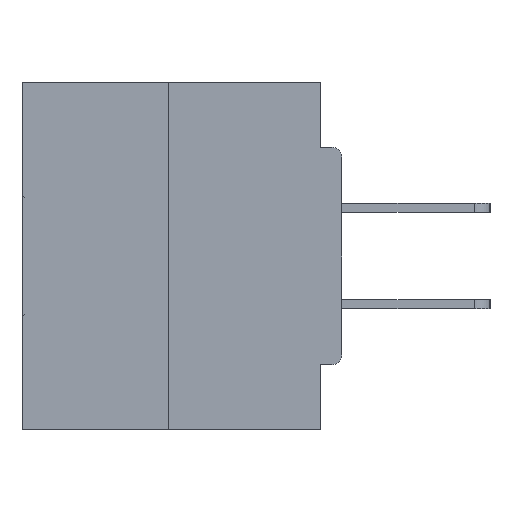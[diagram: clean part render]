
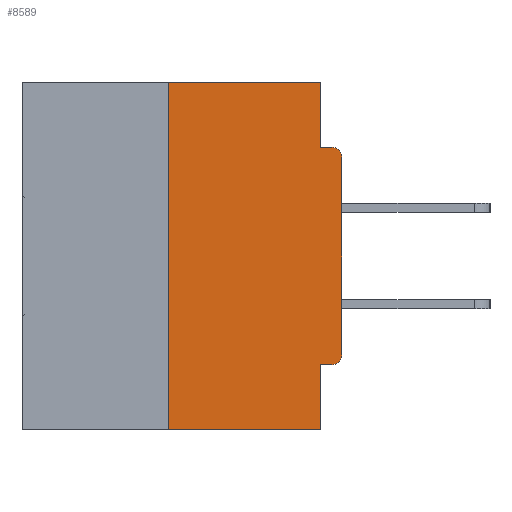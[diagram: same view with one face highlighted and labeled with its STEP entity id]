
A CAD part, left-side view. The second image highlights one B-rep face of the part: STEP entity #8589.
In plain terms, the highlighted planar face has unit normal (-1, 0, 0).
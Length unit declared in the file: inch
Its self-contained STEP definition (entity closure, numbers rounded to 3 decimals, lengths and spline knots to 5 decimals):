
#733 = LINE ( 'NONE', #10267, #17764 ) ;
#764 = VERTEX_POINT ( 'NONE', #37762 ) ;
#1586 = CARTESIAN_POINT ( 'NONE',  ( 0., 0., -0.3915 ) ) ;
#2046 = CARTESIAN_POINT ( 'NONE',  ( 0., 0., -0.0935 ) ) ;
#2396 = ORIENTED_EDGE ( 'NONE', *, *, #37040, .T. ) ;
#2832 = LINE ( 'NONE', #18832, #3875 ) ;
#3875 = VECTOR ( 'NONE', #12178, 39.37008 ) ;
#3882 = ORIENTED_EDGE ( 'NONE', *, *, #20483, .F. ) ;
#5641 = CARTESIAN_POINT ( 'NONE',  ( 0., 0.015, -0.1085 ) ) ;
#5888 = VERTEX_POINT ( 'NONE', #15403 ) ;
#6257 = DIRECTION ( 'NONE',  ( 0., 0., -1. ) ) ;
#7537 = LINE ( 'NONE', #38328, #28983 ) ;
#7588 = VERTEX_POINT ( 'NONE', #38716 ) ;
#7841 = VERTEX_POINT ( 'NONE', #35163 ) ;
#8545 = DIRECTION ( 'NONE',  ( 0., 0., 1. ) ) ;
#8589 = ADVANCED_FACE ( 'NONE', ( #15275 ), #27434, .F. ) ;
#8848 = EDGE_CURVE ( 'NONE', #7841, #5888, #20294, .T. ) ;
#9778 = DIRECTION ( 'NONE',  ( 0., 0., -1. ) ) ;
#10267 = CARTESIAN_POINT ( 'NONE',  ( 0., 0., 0. ) ) ;
#10651 = ORIENTED_EDGE ( 'NONE', *, *, #24445, .F. ) ;
#10843 = ORIENTED_EDGE ( 'NONE', *, *, #22817, .T. ) ;
#11865 = VERTEX_POINT ( 'NONE', #22563 ) ;
#12178 = DIRECTION ( 'NONE',  ( 0., 0., -1. ) ) ;
#12375 = CIRCLE ( 'NONE', #34982, 0.015 ) ;
#12980 = DIRECTION ( 'NONE',  ( 0., 0., -1. ) ) ;
#13214 = ORIENTED_EDGE ( 'NONE', *, *, #31585, .F. ) ;
#13827 = DIRECTION ( 'NONE',  ( 0., -1., 0. ) ) ;
#13880 = EDGE_LOOP ( 'NONE', ( #26750, #13214, #10843, #32011, #3882, #2396, #17291, #15382, #14777, #10651 ) ) ;
#13965 = EDGE_CURVE ( 'NONE', #7588, #19738, #7537, .T. ) ;
#14474 = VECTOR ( 'NONE', #31042, 39.37008 ) ;
#14777 = ORIENTED_EDGE ( 'NONE', *, *, #8848, .F. ) ;
#15275 = FACE_OUTER_BOUND ( 'NONE', #13880, .T. ) ;
#15382 = ORIENTED_EDGE ( 'NONE', *, *, #29497, .T. ) ;
#15403 = CARTESIAN_POINT ( 'NONE',  ( 0., 0.015, -0.0935 ) ) ;
#15843 = LINE ( 'NONE', #34251, #22243 ) ;
#16176 = VERTEX_POINT ( 'NONE', #1586 ) ;
#17291 = ORIENTED_EDGE ( 'NONE', *, *, #23806, .T. ) ;
#17660 = VECTOR ( 'NONE', #36075, 39.37008 ) ;
#17764 = VECTOR ( 'NONE', #31330, 39.37008 ) ;
#18023 = DIRECTION ( 'NONE',  ( 0., 0., -1. ) ) ;
#18832 = CARTESIAN_POINT ( 'NONE',  ( 0., 0.031, -0.5 ) ) ;
#19074 = VECTOR ( 'NONE', #6257, 39.37008 ) ;
#19128 = AXIS2_PLACEMENT_3D ( 'NONE', #5641, #32589, #18023 ) ;
#19738 = VERTEX_POINT ( 'NONE', #21620 ) ;
#20294 = LINE ( 'NONE', #2046, #17660 ) ;
#20327 = CARTESIAN_POINT ( 'NONE',  ( 0., 0.015, -0.4065 ) ) ;
#20483 = EDGE_CURVE ( 'NONE', #27282, #27131, #37099, .T. ) ;
#21620 = CARTESIAN_POINT ( 'NONE',  ( 0., 0.031, 0. ) ) ;
#22094 = CARTESIAN_POINT ( 'NONE',  ( 0., 0.015, -0.3915 ) ) ;
#22243 = VECTOR ( 'NONE', #37493, 39.37008 ) ;
#22563 = CARTESIAN_POINT ( 'NONE',  ( 0., 0., -0.1085 ) ) ;
#22817 = EDGE_CURVE ( 'NONE', #28134, #764, #15843, .T. ) ;
#23041 = VECTOR ( 'NONE', #8545, 39.37008 ) ;
#23806 = EDGE_CURVE ( 'NONE', #16176, #11865, #733, .T. ) ;
#24155 = CARTESIAN_POINT ( 'NONE',  ( 0., 0., -0.4065 ) ) ;
#24445 = EDGE_CURVE ( 'NONE', #19738, #7841, #28368, .T. ) ;
#26099 = DIRECTION ( 'NONE',  ( -1., 0., 0. ) ) ;
#26750 = ORIENTED_EDGE ( 'NONE', *, *, #13965, .F. ) ;
#27131 = VERTEX_POINT ( 'NONE', #38752 ) ;
#27282 = VERTEX_POINT ( 'NONE', #20327 ) ;
#27434 = PLANE ( 'NONE',  #29200 ) ;
#27642 = CARTESIAN_POINT ( 'NONE',  ( 0., 0.46, 0. ) ) ;
#28134 = VERTEX_POINT ( 'NONE', #32930 ) ;
#28368 = LINE ( 'NONE', #30993, #19074 ) ;
#28983 = VECTOR ( 'NONE', #13827, 39.37008 ) ;
#29200 = AXIS2_PLACEMENT_3D ( 'NONE', #27642, #31063, #9778 ) ;
#29497 = EDGE_CURVE ( 'NONE', #11865, #5888, #30796, .T. ) ;
#30796 = CIRCLE ( 'NONE', #19128, 0.015 ) ;
#30993 = CARTESIAN_POINT ( 'NONE',  ( 0., 0.031, 0. ) ) ;
#31042 = DIRECTION ( 'NONE',  ( 0., 1., 0. ) ) ;
#31063 = DIRECTION ( 'NONE',  ( 1., 0., 0. ) ) ;
#31330 = DIRECTION ( 'NONE',  ( 0., 0., 1. ) ) ;
#31585 = EDGE_CURVE ( 'NONE', #28134, #7588, #36299, .T. ) ;
#32011 = ORIENTED_EDGE ( 'NONE', *, *, #35688, .F. ) ;
#32589 = DIRECTION ( 'NONE',  ( -1., 0., 0. ) ) ;
#32930 = CARTESIAN_POINT ( 'NONE',  ( 0., 0.25, -0.5 ) ) ;
#34251 = CARTESIAN_POINT ( 'NONE',  ( 0., 0.46, -0.5 ) ) ;
#34982 = AXIS2_PLACEMENT_3D ( 'NONE', #22094, #26099, #12980 ) ;
#35163 = CARTESIAN_POINT ( 'NONE',  ( 0., 0.031, -0.0935 ) ) ;
#35685 = CARTESIAN_POINT ( 'NONE',  ( 0., 0.25, 0. ) ) ;
#35688 = EDGE_CURVE ( 'NONE', #27131, #764, #2832, .T. ) ;
#36075 = DIRECTION ( 'NONE',  ( 0., -1., 0. ) ) ;
#36299 = LINE ( 'NONE', #35685, #23041 ) ;
#37040 = EDGE_CURVE ( 'NONE', #27282, #16176, #12375, .T. ) ;
#37099 = LINE ( 'NONE', #24155, #14474 ) ;
#37493 = DIRECTION ( 'NONE',  ( 0., -1., 0. ) ) ;
#37762 = CARTESIAN_POINT ( 'NONE',  ( 0., 0.031, -0.5 ) ) ;
#38328 = CARTESIAN_POINT ( 'NONE',  ( 0., 0.46, 0. ) ) ;
#38716 = CARTESIAN_POINT ( 'NONE',  ( 0., 0.25, 0. ) ) ;
#38752 = CARTESIAN_POINT ( 'NONE',  ( 0., 0.031, -0.4065 ) ) ;
